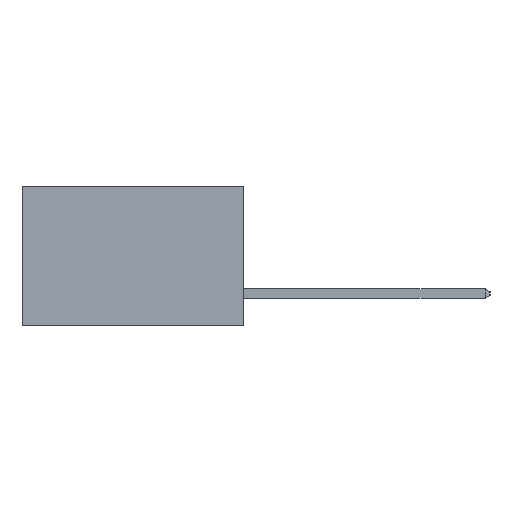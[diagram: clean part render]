
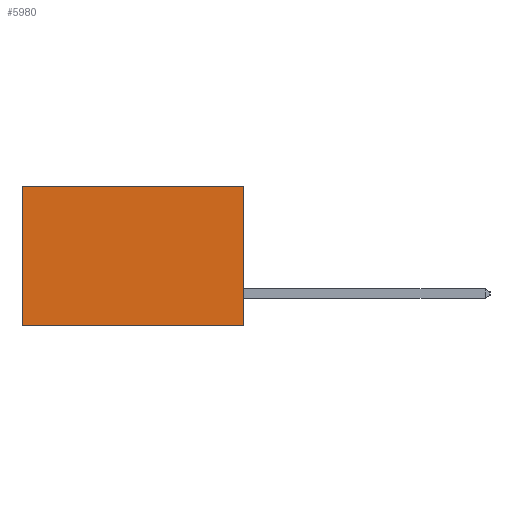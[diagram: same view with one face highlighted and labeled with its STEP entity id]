
A CAD part, left-side view. The second image highlights one B-rep face of the part: STEP entity #5980.
In plain terms, the highlighted planar face has unit normal (-1, 0, 0).
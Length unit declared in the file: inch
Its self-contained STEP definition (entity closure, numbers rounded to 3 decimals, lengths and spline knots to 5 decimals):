
#585 = FACE_OUTER_BOUND ( 'NONE', #6818, .T. ) ;
#808 = EDGE_CURVE ( 'NONE', #7564, #12171, #2427, .T. ) ;
#1056 = LINE ( 'NONE', #11765, #11197 ) ;
#2087 = EDGE_CURVE ( 'NONE', #6473, #7564, #6828, .T. ) ;
#2427 = LINE ( 'NONE', #10645, #4091 ) ;
#3147 = CARTESIAN_POINT ( 'NONE',  ( 0.277, 0.59, -0.37 ) ) ;
#3259 = VECTOR ( 'NONE', #9243, 39.37008 ) ;
#3579 = LINE ( 'NONE', #9603, #3259 ) ;
#3749 = CARTESIAN_POINT ( 'NONE',  ( 0.277, 0., -0.37 ) ) ;
#3905 = EDGE_CURVE ( 'NONE', #6473, #8009, #3579, .T. ) ;
#4091 = VECTOR ( 'NONE', #6297, 39.37008 ) ;
#4408 = DIRECTION ( 'NONE',  ( 0., 0., -1. ) ) ;
#4562 = DIRECTION ( 'NONE',  ( 1., 0., 0. ) ) ;
#4825 = PLANE ( 'NONE',  #7840 ) ;
#5583 = CARTESIAN_POINT ( 'NONE',  ( 0.277, 0., -0.37 ) ) ;
#5889 = ORIENTED_EDGE ( 'NONE', *, *, #808, .T. ) ;
#5894 = ORIENTED_EDGE ( 'NONE', *, *, #6155, .F. ) ;
#5980 = ADVANCED_FACE ( 'NONE', ( #585 ), #4825, .F. ) ;
#6155 = EDGE_CURVE ( 'NONE', #8009, #12171, #1056, .T. ) ;
#6297 = DIRECTION ( 'NONE',  ( 0., 0., -1. ) ) ;
#6473 = VERTEX_POINT ( 'NONE', #7281 ) ;
#6818 = EDGE_LOOP ( 'NONE', ( #5889, #5894, #8773, #9636 ) ) ;
#6828 = LINE ( 'NONE', #12112, #9609 ) ;
#7281 = CARTESIAN_POINT ( 'NONE',  ( 0.277, 0., 0. ) ) ;
#7564 = VERTEX_POINT ( 'NONE', #9632 ) ;
#7840 = AXIS2_PLACEMENT_3D ( 'NONE', #5583, #4562, #4408 ) ;
#8009 = VERTEX_POINT ( 'NONE', #3749 ) ;
#8773 = ORIENTED_EDGE ( 'NONE', *, *, #3905, .F. ) ;
#9243 = DIRECTION ( 'NONE',  ( 0., 0., -1. ) ) ;
#9603 = CARTESIAN_POINT ( 'NONE',  ( 0.277, 0., -0.37 ) ) ;
#9609 = VECTOR ( 'NONE', #12126, 39.37008 ) ;
#9632 = CARTESIAN_POINT ( 'NONE',  ( 0.277, 0.59, 0. ) ) ;
#9636 = ORIENTED_EDGE ( 'NONE', *, *, #2087, .T. ) ;
#10645 = CARTESIAN_POINT ( 'NONE',  ( 0.277, 0.59, -0.37 ) ) ;
#11197 = VECTOR ( 'NONE', #11741, 39.37008 ) ;
#11741 = DIRECTION ( 'NONE',  ( 0., 1., 0. ) ) ;
#11765 = CARTESIAN_POINT ( 'NONE',  ( 0.277, 0., -0.37 ) ) ;
#12112 = CARTESIAN_POINT ( 'NONE',  ( 0.277, 0., 0. ) ) ;
#12126 = DIRECTION ( 'NONE',  ( 0., 1., 0. ) ) ;
#12171 = VERTEX_POINT ( 'NONE', #3147 ) ;
